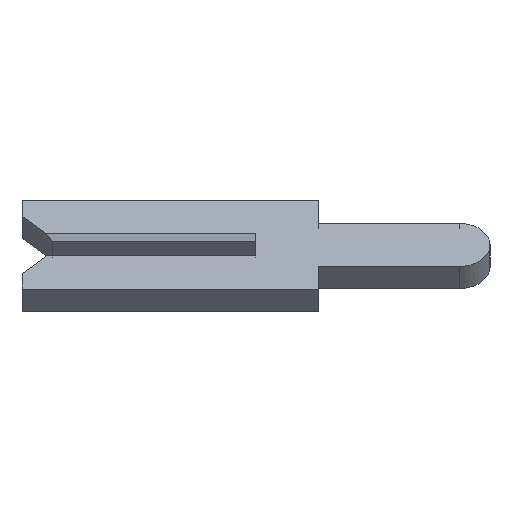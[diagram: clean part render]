
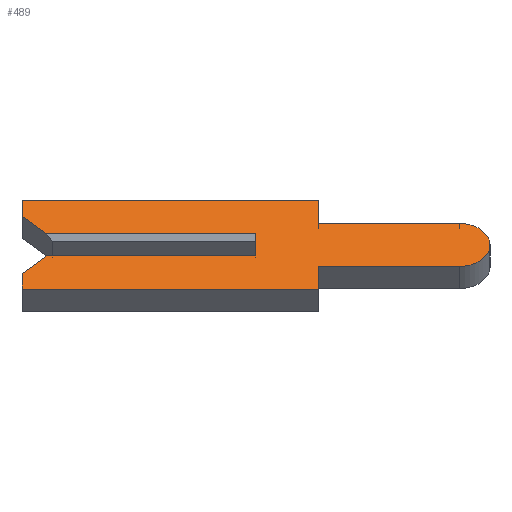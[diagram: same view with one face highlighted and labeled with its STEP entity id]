
A CAD part, left-side view. The second image highlights one B-rep face of the part: STEP entity #489.
In plain terms, the highlighted face is planar.
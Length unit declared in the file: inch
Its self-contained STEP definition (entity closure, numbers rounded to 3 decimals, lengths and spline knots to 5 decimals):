
#9 = EDGE_CURVE ( 'NONE', #615, #668, #910, .T. ) ;
#32 = AXIS2_PLACEMENT_3D ( 'NONE', #190, #362, #353 ) ;
#36 = VERTEX_POINT ( 'NONE', #327 ) ;
#39 = VECTOR ( 'NONE', #566, 39.37008 ) ;
#53 = CARTESIAN_POINT ( 'NONE',  ( -0.01, -0.1305, -0.01 ) ) ;
#61 = VERTEX_POINT ( 'NONE', #144 ) ;
#73 = ORIENTED_EDGE ( 'NONE', *, *, #791, .F. ) ;
#75 = CARTESIAN_POINT ( 'NONE',  ( -0.01, 0., -0.01 ) ) ;
#93 = VECTOR ( 'NONE', #673, 39.37008 ) ;
#100 = CARTESIAN_POINT ( 'NONE',  ( -0.01, 0.15, 0.04 ) ) ;
#102 = VERTEX_POINT ( 'NONE', #1005 ) ;
#105 = VERTEX_POINT ( 'NONE', #1090 ) ;
#112 = CARTESIAN_POINT ( 'NONE',  ( -0.01, 0.15, 0.01 ) ) ;
#114 = EDGE_CURVE ( 'NONE', #105, #318, #509, .T. ) ;
#118 = VECTOR ( 'NONE', #862, 39.37008 ) ;
#120 = EDGE_CURVE ( 'NONE', #293, #105, #779, .T. ) ;
#122 = LINE ( 'NONE', #829, #149 ) ;
#123 = CARTESIAN_POINT ( 'NONE',  ( -0.01, -0.04, -0.04 ) ) ;
#124 = ORIENTED_EDGE ( 'NONE', *, *, #520, .F. ) ;
#141 = LINE ( 'NONE', #847, #517 ) ;
#144 = CARTESIAN_POINT ( 'NONE',  ( -0.01, -0.04, 0.0195 ) ) ;
#149 = VECTOR ( 'NONE', #1010, 39.37008 ) ;
#156 = VERTEX_POINT ( 'NONE', #413 ) ;
#175 = EDGE_CURVE ( 'NONE', #61, #266, #122, .T. ) ;
#190 = CARTESIAN_POINT ( 'NONE',  ( -0.01, -0.1305, 0. ) ) ;
#191 = ORIENTED_EDGE ( 'NONE', *, *, #175, .F. ) ;
#198 = CARTESIAN_POINT ( 'NONE',  ( -0.01, 0.15, 0.04 ) ) ;
#219 = CARTESIAN_POINT ( 'NONE',  ( -0.01, 0., 0.0065 ) ) ;
#238 = ORIENTED_EDGE ( 'NONE', *, *, #1065, .F. ) ;
#246 = EDGE_CURVE ( 'NONE', #102, #615, #393, .T. ) ;
#248 = CARTESIAN_POINT ( 'NONE',  ( -0.01, 0.15, -0.04 ) ) ;
#262 = VERTEX_POINT ( 'NONE', #248 ) ;
#266 = VERTEX_POINT ( 'NONE', #943 ) ;
#270 = CARTESIAN_POINT ( 'NONE',  ( -0.01, -0.04, -0.0195 ) ) ;
#293 = VERTEX_POINT ( 'NONE', #765 ) ;
#307 = EDGE_CURVE ( 'NONE', #721, #156, #141, .T. ) ;
#314 = CARTESIAN_POINT ( 'NONE',  ( -0.01, 0.15, -0.026 ) ) ;
#317 = DIRECTION ( 'NONE',  ( 0., -0.707, 0.707 ) ) ;
#318 = VERTEX_POINT ( 'NONE', #75 ) ;
#324 = ORIENTED_EDGE ( 'NONE', *, *, #928, .F. ) ;
#327 = CARTESIAN_POINT ( 'NONE',  ( -0.01, 0., 0.01 ) ) ;
#330 = DIRECTION ( 'NONE',  ( 0., -1., 0. ) ) ;
#353 = DIRECTION ( 'NONE',  ( 0., 0., -1. ) ) ;
#362 = DIRECTION ( 'NONE',  ( 1., 0., 0. ) ) ;
#375 = LINE ( 'NONE', #433, #1089 ) ;
#376 = CARTESIAN_POINT ( 'NONE',  ( -0.01, 0.134, 0.01 ) ) ;
#386 = ORIENTED_EDGE ( 'NONE', *, *, #120, .F. ) ;
#393 = LINE ( 'NONE', #778, #1063 ) ;
#413 = CARTESIAN_POINT ( 'NONE',  ( -0.01, 0.15, 0.026 ) ) ;
#433 = CARTESIAN_POINT ( 'NONE',  ( -0.01, 0.15, -0.04 ) ) ;
#456 = EDGE_CURVE ( 'NONE', #668, #262, #375, .T. ) ;
#469 = EDGE_CURVE ( 'NONE', #676, #61, #845, .T. ) ;
#482 = VECTOR ( 'NONE', #697, 39.37008 ) ;
#489 = ADVANCED_FACE ( 'NONE', ( #741 ), #538, .F. ) ;
#509 = LINE ( 'NONE', #53, #683 ) ;
#517 = VECTOR ( 'NONE', #843, 39.37008 ) ;
#520 = EDGE_CURVE ( 'NONE', #536, #676, #848, .T. ) ;
#536 = VERTEX_POINT ( 'NONE', #198 ) ;
#538 = PLANE ( 'NONE',  #32 ) ;
#551 = VECTOR ( 'NONE', #317, 39.37008 ) ;
#561 = EDGE_CURVE ( 'NONE', #721, #36, #715, .T. ) ;
#566 = DIRECTION ( 'NONE',  ( 0., 0., 1. ) ) ;
#592 = AXIS2_PLACEMENT_3D ( 'NONE', #901, #651, #1085 ) ;
#596 = VECTOR ( 'NONE', #960, 39.37008 ) ;
#615 = VERTEX_POINT ( 'NONE', #270 ) ;
#618 = ORIENTED_EDGE ( 'NONE', *, *, #114, .F. ) ;
#634 = ORIENTED_EDGE ( 'NONE', *, *, #1059, .F. ) ;
#646 = DIRECTION ( 'NONE',  ( 0., 0., 1. ) ) ;
#648 = ORIENTED_EDGE ( 'NONE', *, *, #561, .T. ) ;
#651 = DIRECTION ( 'NONE',  ( 1., 0., 0. ) ) ;
#668 = VERTEX_POINT ( 'NONE', #123 ) ;
#670 = ORIENTED_EDGE ( 'NONE', *, *, #456, .F. ) ;
#673 = DIRECTION ( 'NONE',  ( 0., 0., -1. ) ) ;
#676 = VERTEX_POINT ( 'NONE', #1075 ) ;
#683 = VECTOR ( 'NONE', #330, 39.37008 ) ;
#690 = DIRECTION ( 'NONE',  ( 0., 1., 0. ) ) ;
#697 = DIRECTION ( 'NONE',  ( 0., -1., 0. ) ) ;
#715 = LINE ( 'NONE', #112, #482 ) ;
#721 = VERTEX_POINT ( 'NONE', #376 ) ;
#731 = LINE ( 'NONE', #314, #39 ) ;
#741 = FACE_OUTER_BOUND ( 'NONE', #835, .T. ) ;
#756 = ORIENTED_EDGE ( 'NONE', *, *, #246, .F. ) ;
#765 = CARTESIAN_POINT ( 'NONE',  ( -0.01, 0.15, -0.026 ) ) ;
#778 = CARTESIAN_POINT ( 'NONE',  ( -0.01, -0.04, -0.0195 ) ) ;
#779 = LINE ( 'NONE', #822, #551 ) ;
#791 = EDGE_CURVE ( 'NONE', #156, #536, #947, .T. ) ;
#822 = CARTESIAN_POINT ( 'NONE',  ( -0.01, 0.1305, -0.0065 ) ) ;
#829 = CARTESIAN_POINT ( 'NONE',  ( -0.01, -0.04, 0.0195 ) ) ;
#835 = EDGE_LOOP ( 'NONE', ( #648, #238, #618, #386, #634, #670, #978, #756, #324, #191, #999, #124, #73, #922 ) ) ;
#843 = DIRECTION ( 'NONE',  ( 0., 0.707, 0.707 ) ) ;
#845 = LINE ( 'NONE', #950, #596 ) ;
#847 = CARTESIAN_POINT ( 'NONE',  ( -0.01, 0.1305, 0.0065 ) ) ;
#848 = LINE ( 'NONE', #100, #118 ) ;
#853 = CIRCLE ( 'NONE', #592, 0.0195 ) ;
#862 = DIRECTION ( 'NONE',  ( 0., -1., 0. ) ) ;
#868 = LINE ( 'NONE', #219, #1040 ) ;
#889 = DIRECTION ( 'NONE',  ( 0., 0., 1. ) ) ;
#901 = CARTESIAN_POINT ( 'NONE',  ( -0.01, -0.1305, 0. ) ) ;
#909 = CARTESIAN_POINT ( 'NONE',  ( -0.01, -0.04, -0.04 ) ) ;
#910 = LINE ( 'NONE', #909, #93 ) ;
#922 = ORIENTED_EDGE ( 'NONE', *, *, #307, .F. ) ;
#928 = EDGE_CURVE ( 'NONE', #266, #102, #853, .T. ) ;
#943 = CARTESIAN_POINT ( 'NONE',  ( -0.01, -0.1305, 0.0195 ) ) ;
#947 = LINE ( 'NONE', #973, #976 ) ;
#950 = CARTESIAN_POINT ( 'NONE',  ( -0.01, -0.04, 0.04 ) ) ;
#960 = DIRECTION ( 'NONE',  ( 0., 0., -1. ) ) ;
#973 = CARTESIAN_POINT ( 'NONE',  ( -0.01, 0.15, 0.026 ) ) ;
#976 = VECTOR ( 'NONE', #889, 39.37008 ) ;
#978 = ORIENTED_EDGE ( 'NONE', *, *, #9, .F. ) ;
#999 = ORIENTED_EDGE ( 'NONE', *, *, #469, .F. ) ;
#1005 = CARTESIAN_POINT ( 'NONE',  ( -0.01, -0.1305, -0.0195 ) ) ;
#1010 = DIRECTION ( 'NONE',  ( 0., -1., 0. ) ) ;
#1040 = VECTOR ( 'NONE', #646, 39.37008 ) ;
#1048 = DIRECTION ( 'NONE',  ( 0., 1., 0. ) ) ;
#1059 = EDGE_CURVE ( 'NONE', #262, #293, #731, .T. ) ;
#1063 = VECTOR ( 'NONE', #690, 39.37008 ) ;
#1065 = EDGE_CURVE ( 'NONE', #318, #36, #868, .T. ) ;
#1075 = CARTESIAN_POINT ( 'NONE',  ( -0.01, -0.04, 0.04 ) ) ;
#1085 = DIRECTION ( 'NONE',  ( 0., 0., -1. ) ) ;
#1089 = VECTOR ( 'NONE', #1048, 39.37008 ) ;
#1090 = CARTESIAN_POINT ( 'NONE',  ( -0.01, 0.134, -0.01 ) ) ;
